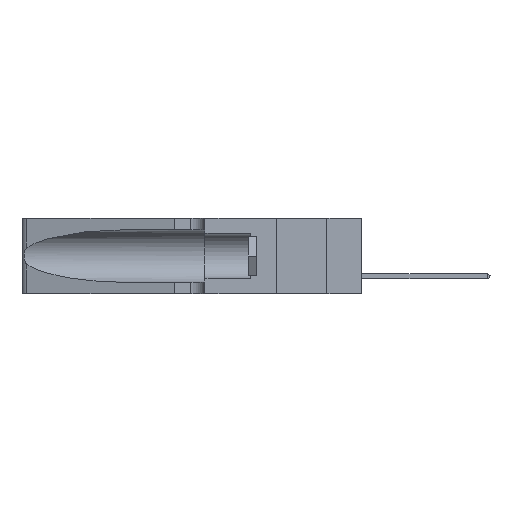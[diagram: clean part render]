
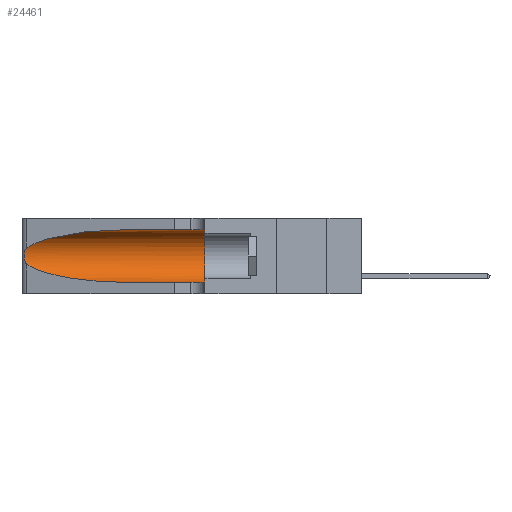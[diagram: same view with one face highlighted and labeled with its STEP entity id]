
A CAD part, left-side view. The second image highlights one B-rep face of the part: STEP entity #24461.
In plain terms, the highlighted cylindrical face has radius 3.308 mm (diameter 6.617 mm), a partial arc.
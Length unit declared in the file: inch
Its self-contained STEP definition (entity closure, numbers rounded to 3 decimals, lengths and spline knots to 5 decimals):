
#443 = AXIS2_PLACEMENT_3D ( 'NONE', #16417, #12379, #14578 ) ;
#1044 = CARTESIAN_POINT ( 'NONE',  ( 0.1305, 1.61858, 0.185 ) ) ;
#1136 = DIRECTION ( 'NONE',  ( 0., -1., 0. ) ) ;
#1500 = B_SPLINE_CURVE_WITH_KNOTS ( 'NONE', 3,
 ( #19588, #30583, #5885, #11752, #22439, #27650, #3602, #33414, #6353, #25027, #9111, #25144, #3236, #6125 ),
 .UNSPECIFIED., .F., .F.,
 ( 4, 2, 2, 2, 2, 2, 4 ),
 ( 0., 0.00027, 0.00053, 0.00107, 0.0016, 0.00187, 0.00214 ),
 .UNSPECIFIED. ) ;
#2187 = EDGE_LOOP ( 'NONE', ( #5293, #26537, #6208, #29658, #19890, #30393 ) ) ;
#2809 = VERTEX_POINT ( 'NONE', #2892 ) ;
#2892 = CARTESIAN_POINT ( 'NONE',  ( 0.1305, 0.35, 0.31525 ) ) ;
#3236 = CARTESIAN_POINT ( 'NONE',  ( 0.25555, 1.22993, 0.14849 ) ) ;
#3602 = CARTESIAN_POINT ( 'NONE',  ( 0.26075, 1.23896, 0.19203 ) ) ;
#3863 = DIRECTION ( 'NONE',  ( 0., -1., 0. ) ) ;
#3963 = CARTESIAN_POINT ( 'NONE',  ( 0.1305, 1.61858, 0.05475 ) ) ;
#4217 = FACE_OUTER_BOUND ( 'NONE', #2187, .T. ) ;
#5242 =( BOUNDED_CURVE ( )  B_SPLINE_CURVE ( 3, ( #32713, #27428, #6131, #8990 ),
 .UNSPECIFIED., .F., .F. ) 
 B_SPLINE_CURVE_WITH_KNOTS ( ( 4, 4 ),
 ( 1.5708, 2.84003 ),
 .UNSPECIFIED. ) 
 CURVE ( )  GEOMETRIC_REPRESENTATION_ITEM ( )  RATIONAL_B_SPLINE_CURVE ( ( 1., 0.87, 0.87, 1. ) ) 
 REPRESENTATION_ITEM ( '' )  );
#5293 = ORIENTED_EDGE ( 'NONE', *, *, #9756, .T. ) ;
#5383 = VERTEX_POINT ( 'NONE', #24424 ) ;
#5885 = CARTESIAN_POINT ( 'NONE',  ( 0.25639, 1.23184, 0.21858 ) ) ;
#6125 = CARTESIAN_POINT ( 'NONE',  ( 0.25487, 1.22718, 0.14631 ) ) ;
#6131 = CARTESIAN_POINT ( 'NONE',  ( 0.2373, 1.15595, 0.28018 ) ) ;
#6208 = ORIENTED_EDGE ( 'NONE', *, *, #30717, .T. ) ;
#6353 = CARTESIAN_POINT ( 'NONE',  ( 0.26017, 1.23833, 0.17102 ) ) ;
#6786 = LINE ( 'NONE', #23343, #8493 ) ;
#8493 = VECTOR ( 'NONE', #20751, 39.37008 ) ;
#8990 = CARTESIAN_POINT ( 'NONE',  ( 0.25487, 1.22718, 0.22369 ) ) ;
#9111 = CARTESIAN_POINT ( 'NONE',  ( 0.25789, 1.23486, 0.15765 ) ) ;
#9756 = EDGE_CURVE ( 'NONE', #23086, #5383, #5242, .T. ) ;
#9878 = CARTESIAN_POINT ( 'NONE',  ( 0.1305, 0.72297, 0.31525 ) ) ;
#11752 = CARTESIAN_POINT ( 'NONE',  ( 0.25787, 1.23484, 0.2124 ) ) ;
#12379 = DIRECTION ( 'NONE',  ( 0., 1., 0. ) ) ;
#14578 = DIRECTION ( 'NONE',  ( 0., 0., 1. ) ) ;
#15277 = CARTESIAN_POINT ( 'NONE',  ( 0.25487, 1.22718, 0.14631 ) ) ;
#15491 = EDGE_CURVE ( 'NONE', #23086, #2809, #6786, .T. ) ;
#16417 = CARTESIAN_POINT ( 'NONE',  ( 0.1305, 0.35, 0.185 ) ) ;
#18754 = CYLINDRICAL_SURFACE ( 'NONE', #24392, 0.13025 ) ;
#19020 = VECTOR ( 'NONE', #1136, 39.37008 ) ;
#19588 = CARTESIAN_POINT ( 'NONE',  ( 0.25487, 1.22718, 0.22369 ) ) ;
#19890 = ORIENTED_EDGE ( 'NONE', *, *, #24982, .F. ) ;
#20751 = DIRECTION ( 'NONE',  ( 0., -1., 0. ) ) ;
#20759 = CARTESIAN_POINT ( 'NONE',  ( 0.2373, 1.15595, 0.08982 ) ) ;
#21203 = EDGE_CURVE ( 'NONE', #5383, #23257, #1500, .T. ) ;
#21405 = EDGE_CURVE ( 'NONE', #30524, #31679, #32538, .T. ) ;
#21775 = CARTESIAN_POINT ( 'NONE',  ( 0.1305, 0.35, 0.05475 ) ) ;
#22439 = CARTESIAN_POINT ( 'NONE',  ( 0.25854, 1.2359, 0.20912 ) ) ;
#23086 = VERTEX_POINT ( 'NONE', #9878 ) ;
#23257 = VERTEX_POINT ( 'NONE', #26599 ) ;
#23343 = CARTESIAN_POINT ( 'NONE',  ( 0.1305, 1.61858, 0.31525 ) ) ;
#24392 = AXIS2_PLACEMENT_3D ( 'NONE', #1044, #3863, #30492 ) ;
#24424 = CARTESIAN_POINT ( 'NONE',  ( 0.25487, 1.22718, 0.22369 ) ) ;
#24461 = ADVANCED_FACE ( 'NONE', ( #4217 ), #18754, .F. ) ;
#24982 = EDGE_CURVE ( 'NONE', #2809, #31679, #34764, .T. ) ;
#25027 = CARTESIAN_POINT ( 'NONE',  ( 0.25856, 1.23593, 0.16098 ) ) ;
#25144 = CARTESIAN_POINT ( 'NONE',  ( 0.25639, 1.23186, 0.15144 ) ) ;
#25274 =( BOUNDED_CURVE ( )  B_SPLINE_CURVE ( 3, ( #15277, #20759, #26198, #28580 ),
 .UNSPECIFIED., .F., .F. ) 
 B_SPLINE_CURVE_WITH_KNOTS ( ( 4, 4 ),
 ( 3.44316, 4.71239 ),
 .UNSPECIFIED. ) 
 CURVE ( )  GEOMETRIC_REPRESENTATION_ITEM ( )  RATIONAL_B_SPLINE_CURVE ( ( 1., 0.87, 0.87, 1. ) ) 
 REPRESENTATION_ITEM ( '' )  );
#26198 = CARTESIAN_POINT ( 'NONE',  ( 0.18966, 0.96281, 0.05475 ) ) ;
#26537 = ORIENTED_EDGE ( 'NONE', *, *, #21203, .T. ) ;
#26599 = CARTESIAN_POINT ( 'NONE',  ( 0.25487, 1.22718, 0.14631 ) ) ;
#27428 = CARTESIAN_POINT ( 'NONE',  ( 0.18966, 0.96281, 0.31525 ) ) ;
#27650 = CARTESIAN_POINT ( 'NONE',  ( 0.26018, 1.23835, 0.19895 ) ) ;
#28580 = CARTESIAN_POINT ( 'NONE',  ( 0.1305, 0.72297, 0.05475 ) ) ;
#29658 = ORIENTED_EDGE ( 'NONE', *, *, #21405, .T. ) ;
#30393 = ORIENTED_EDGE ( 'NONE', *, *, #15491, .F. ) ;
#30492 = DIRECTION ( 'NONE',  ( 0., 0., -1. ) ) ;
#30524 = VERTEX_POINT ( 'NONE', #30564 ) ;
#30564 = CARTESIAN_POINT ( 'NONE',  ( 0.1305, 0.72297, 0.05475 ) ) ;
#30583 = CARTESIAN_POINT ( 'NONE',  ( 0.25555, 1.22994, 0.2215 ) ) ;
#30717 = EDGE_CURVE ( 'NONE', #23257, #30524, #25274, .T. ) ;
#31679 = VERTEX_POINT ( 'NONE', #21775 ) ;
#32538 = LINE ( 'NONE', #3963, #19020 ) ;
#32713 = CARTESIAN_POINT ( 'NONE',  ( 0.1305, 0.72297, 0.31525 ) ) ;
#33414 = CARTESIAN_POINT ( 'NONE',  ( 0.26075, 1.23896, 0.178 ) ) ;
#34764 = CIRCLE ( 'NONE', #443, 0.13025 ) ;
